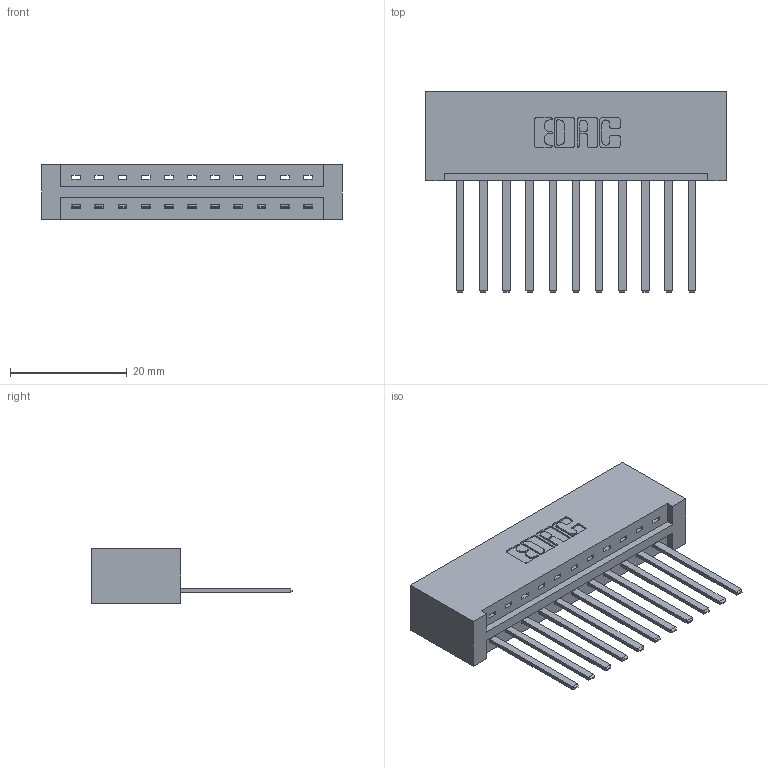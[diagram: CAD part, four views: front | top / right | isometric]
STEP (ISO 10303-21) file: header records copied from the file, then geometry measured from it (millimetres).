
FILE_DESCRIPTION (( 'STEP AP203' ), '1' );
FILE_NAME ('387-011-544-101.STEP', '2019-10-02T12:33:20', ( '' ), ( '' ), 'SwSTEP 2.0', 'SolidWorks 2016', '' );
FILE_SCHEMA (( 'CONFIG_CONTROL_DESIGN' ));
Length unit declared in the file: inch
Products named in the file (3): 387-011-544-101; 337 Part_No Mounting Lugs; 345-292-001_345-293-144
Assembly tree (12 placements, depth 2):
  387-011-544-101
    337 Part_No Mounting Lugs
    345-292-001_345-293-144  x11
Bounding box: 51.46 x 34.3 x 9.4 mm (x, y, z)
Volume: 5826.6 mm3; surface area: 6249.4 mm2
Topology: 12 solids, 12 shells, 722 faces, 2157 edges, 1422 vertices
Faces by surface type: plane 528, cylinder 194
Entity records: 11725 total; most frequent: CARTESIAN_POINT 2047, ORIENTED_EDGE 1994, DIRECTION 1775, EDGE_CURVE 997, VECTOR 881, LINE 881, VERTEX_POINT 662, AXIS2_PLACEMENT_3D 447
